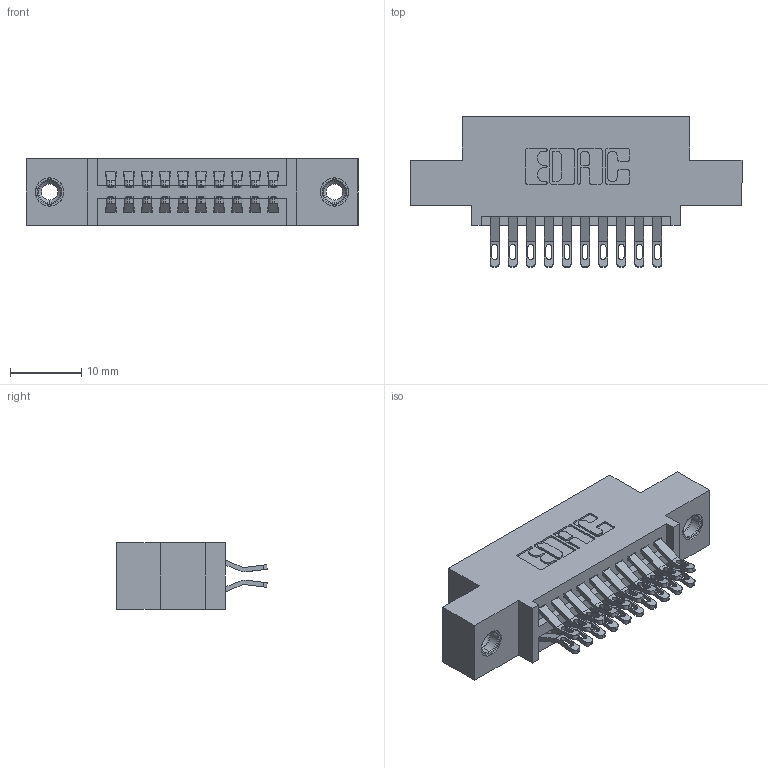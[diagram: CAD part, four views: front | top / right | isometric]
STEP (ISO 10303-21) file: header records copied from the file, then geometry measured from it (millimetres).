
FILE_DESCRIPTION (( 'STEP AP203' ), '1' );
FILE_NAME ('345-020-555-508.STEP', '2019-10-27T09:03:40', ( '' ), ( '' ), 'SwSTEP 2.0', 'SolidWorks 2016', '' );
FILE_SCHEMA (( 'CONFIG_CONTROL_DESIGN' ));
Length unit declared in the file: inch
Products named in the file (4): 345-020-555-508; 345-250-001_345-250-003-102; 345-292-001_555 Tail; 345 Part_0.110 Offset - 0.156 Dia-TI
Assembly tree (23 placements, depth 2):
  345-020-555-508
    345 Part_0.110 Offset - 0.156 Dia-TI
    345-292-001_555 Tail  x20
    345-250-001_345-250-003-102  x2
Bounding box: 46.61 x 21.13 x 9.4 mm (x, y, z)
Volume: 4208.7 mm3; surface area: 5909.5 mm2
Topology: 23 solids, 23 shells, 1310 faces, 4029 edges, 2678 vertices
Faces by surface type: plane 736, cylinder 558, cone 12, torus 4
Entity records: 13798 total; most frequent: CARTESIAN_POINT 2361, ORIENTED_EDGE 2258, DIRECTION 2115, EDGE_CURVE 1129, LINE 917, VECTOR 917, VERTEX_POINT 748, AXIS2_PLACEMENT_3D 599
